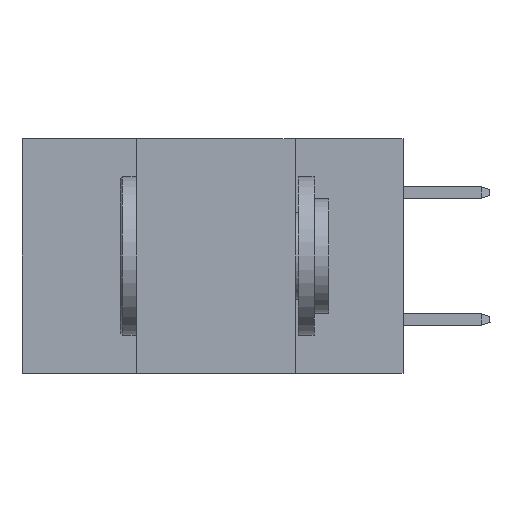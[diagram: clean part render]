
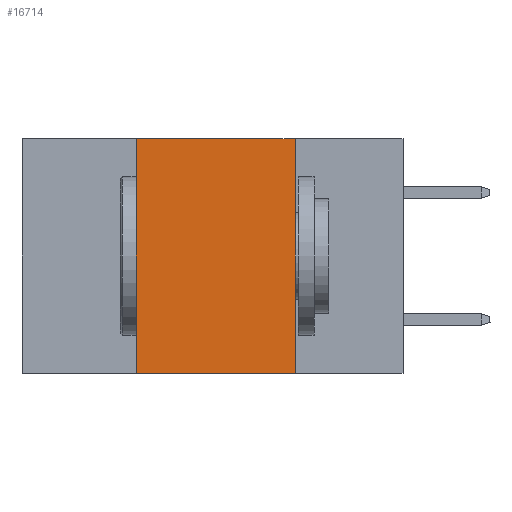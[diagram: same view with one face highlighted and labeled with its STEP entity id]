
A CAD part, left-side view. The second image highlights one B-rep face of the part: STEP entity #16714.
In plain terms, the highlighted planar face has unit normal (-1, 0, 0).
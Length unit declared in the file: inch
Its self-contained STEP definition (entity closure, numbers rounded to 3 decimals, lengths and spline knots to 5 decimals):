
#490 = LINE ( 'NONE', #22811, #14273 ) ;
#705 = DIRECTION ( 'NONE',  ( 1., 0., 0. ) ) ;
#988 = CARTESIAN_POINT ( 'NONE',  ( 0., 0.6, 0. ) ) ;
#1622 = ORIENTED_EDGE ( 'NONE', *, *, #22077, .F. ) ;
#2781 = DIRECTION ( 'NONE',  ( 0., 0., -1. ) ) ;
#3938 = ORIENTED_EDGE ( 'NONE', *, *, #20943, .F. ) ;
#4726 = DIRECTION ( 'NONE',  ( 0., -1., 0. ) ) ;
#5958 = CARTESIAN_POINT ( 'NONE',  ( 0., 0.17, -0.37 ) ) ;
#6388 = VECTOR ( 'NONE', #13022, 39.37008 ) ;
#7152 = EDGE_CURVE ( 'NONE', #8226, #22225, #21096, .T. ) ;
#8226 = VERTEX_POINT ( 'NONE', #12502 ) ;
#8655 = VERTEX_POINT ( 'NONE', #10135 ) ;
#8928 = DIRECTION ( 'NONE',  ( 0., 0., 1. ) ) ;
#9125 = LINE ( 'NONE', #988, #9830 ) ;
#9152 = ORIENTED_EDGE ( 'NONE', *, *, #7152, .F. ) ;
#9284 = CARTESIAN_POINT ( 'NONE',  ( 0., 0.42, 0. ) ) ;
#9830 = VECTOR ( 'NONE', #4726, 39.37008 ) ;
#10135 = CARTESIAN_POINT ( 'NONE',  ( 0., 0.42, -0.37 ) ) ;
#12486 = DIRECTION ( 'NONE',  ( 0., 0., -1. ) ) ;
#12502 = CARTESIAN_POINT ( 'NONE',  ( 0., 0.17, 0. ) ) ;
#13022 = DIRECTION ( 'NONE',  ( 0., -1., 0. ) ) ;
#13129 = CARTESIAN_POINT ( 'NONE',  ( 0., 0.6, 0. ) ) ;
#14273 = VECTOR ( 'NONE', #8928, 39.37008 ) ;
#14818 = VECTOR ( 'NONE', #12486, 39.37008 ) ;
#16431 = AXIS2_PLACEMENT_3D ( 'NONE', #13129, #705, #2781 ) ;
#16714 = ADVANCED_FACE ( 'NONE', ( #25874 ), #17312, .F. ) ;
#17312 = PLANE ( 'NONE',  #16431 ) ;
#18716 = EDGE_LOOP ( 'NONE', ( #9152, #1622, #3938, #23003 ) ) ;
#19907 = VERTEX_POINT ( 'NONE', #9284 ) ;
#20943 = EDGE_CURVE ( 'NONE', #8655, #19907, #490, .T. ) ;
#21096 = LINE ( 'NONE', #22880, #14818 ) ;
#21365 = CARTESIAN_POINT ( 'NONE',  ( 0., 0.6, -0.37 ) ) ;
#21400 = EDGE_CURVE ( 'NONE', #8655, #22225, #25374, .T. ) ;
#22077 = EDGE_CURVE ( 'NONE', #19907, #8226, #9125, .T. ) ;
#22225 = VERTEX_POINT ( 'NONE', #5958 ) ;
#22811 = CARTESIAN_POINT ( 'NONE',  ( 0., 0.42, 0. ) ) ;
#22880 = CARTESIAN_POINT ( 'NONE',  ( 0., 0.17, 0. ) ) ;
#23003 = ORIENTED_EDGE ( 'NONE', *, *, #21400, .T. ) ;
#25374 = LINE ( 'NONE', #21365, #6388 ) ;
#25874 = FACE_OUTER_BOUND ( 'NONE', #18716, .T. ) ;
